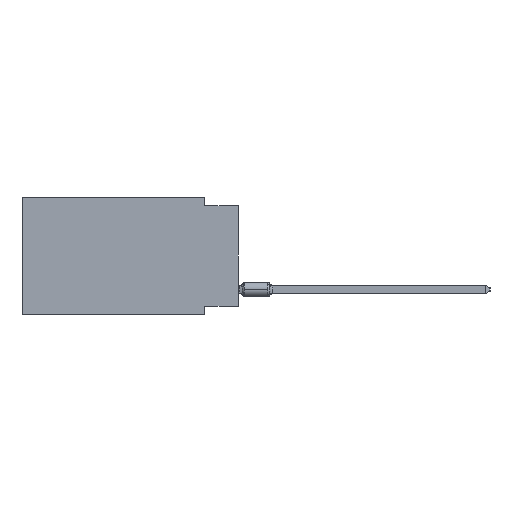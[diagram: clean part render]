
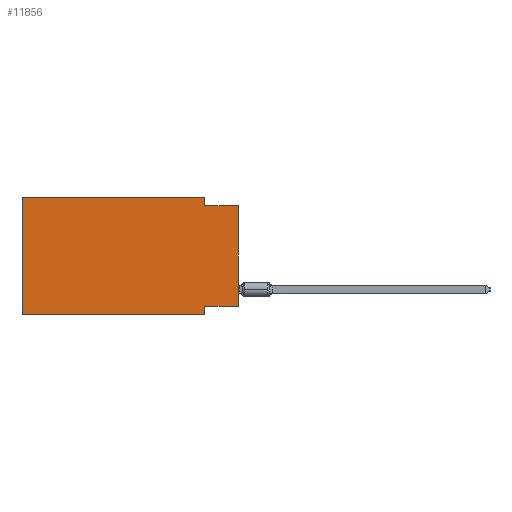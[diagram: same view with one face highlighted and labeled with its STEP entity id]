
A CAD part, left-side view. The second image highlights one B-rep face of the part: STEP entity #11856.
In plain terms, the highlighted planar face has unit normal (-1, 0, 0).
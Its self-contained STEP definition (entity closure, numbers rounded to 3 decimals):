
#1014 = EDGE_CURVE ( 'NONE', #4075, #43226, #54936, .T. ) ;
#1530 = CARTESIAN_POINT ( 'NONE',  ( 0., 2.54, -0.635 ) ) ;
#3191 = CARTESIAN_POINT ( 'NONE',  ( 0., 2.54, -8.255 ) ) ;
#4075 = VERTEX_POINT ( 'NONE', #3191 ) ;
#4749 = DIRECTION ( 'NONE',  ( 0., -1., 0. ) ) ;
#4871 = VECTOR ( 'NONE', #45037, 1000. ) ;
#9013 = VERTEX_POINT ( 'NONE', #46708 ) ;
#9141 = VERTEX_POINT ( 'NONE', #58113 ) ;
#9778 = LINE ( 'NONE', #30232, #64636 ) ;
#10782 = LINE ( 'NONE', #36605, #29411 ) ;
#11094 = DIRECTION ( 'NONE',  ( 0., 1., 0. ) ) ;
#11856 = ADVANCED_FACE ( 'NONE', ( #58854 ), #63882, .F. ) ;
#12960 = ORIENTED_EDGE ( 'NONE', *, *, #26854, .F. ) ;
#14326 = CARTESIAN_POINT ( 'NONE',  ( 0., 2.54, 0. ) ) ;
#17411 = ORIENTED_EDGE ( 'NONE', *, *, #57949, .T. ) ;
#19886 = AXIS2_PLACEMENT_3D ( 'NONE', #28637, #33326, #22628 ) ;
#19986 = LINE ( 'NONE', #25047, #54908 ) ;
#22628 = DIRECTION ( 'NONE',  ( 0., 0., -1. ) ) ;
#22693 = CARTESIAN_POINT ( 'NONE',  ( 0., 16.383, 0. ) ) ;
#24051 = ORIENTED_EDGE ( 'NONE', *, *, #45005, .F. ) ;
#25047 = CARTESIAN_POINT ( 'NONE',  ( 0., 0., -0.635 ) ) ;
#26339 = ORIENTED_EDGE ( 'NONE', *, *, #48039, .T. ) ;
#26854 = EDGE_CURVE ( 'NONE', #54475, #36489, #34770, .T. ) ;
#28362 = ORIENTED_EDGE ( 'NONE', *, *, #33851, .F. ) ;
#28637 = CARTESIAN_POINT ( 'NONE',  ( 0., 16.383, 0. ) ) ;
#29134 = EDGE_LOOP ( 'NONE', ( #26339, #41479, #12960, #24051, #28362, #17411, #55665, #57179 ) ) ;
#29411 = VECTOR ( 'NONE', #46338, 1000. ) ;
#30232 = CARTESIAN_POINT ( 'NONE',  ( 0., 16.383, 0. ) ) ;
#30508 = CARTESIAN_POINT ( 'NONE',  ( 0., 2.54, 0. ) ) ;
#31730 = LINE ( 'NONE', #52192, #57938 ) ;
#32688 = VERTEX_POINT ( 'NONE', #63521 ) ;
#33326 = DIRECTION ( 'NONE',  ( 1., 0., 0. ) ) ;
#33851 = EDGE_CURVE ( 'NONE', #9013, #9141, #39337, .T. ) ;
#34770 = LINE ( 'NONE', #14326, #40556 ) ;
#36489 = VERTEX_POINT ( 'NONE', #1530 ) ;
#36605 = CARTESIAN_POINT ( 'NONE',  ( 0., 0., 0. ) ) ;
#39337 = LINE ( 'NONE', #22693, #4871 ) ;
#40556 = VECTOR ( 'NONE', #42609, 1000. ) ;
#41479 = ORIENTED_EDGE ( 'NONE', *, *, #62569, .F. ) ;
#41804 = CARTESIAN_POINT ( 'NONE',  ( 0., 2.54, -8.89 ) ) ;
#42609 = DIRECTION ( 'NONE',  ( 0., 0., -1. ) ) ;
#43226 = VERTEX_POINT ( 'NONE', #41804 ) ;
#45005 = EDGE_CURVE ( 'NONE', #9141, #54475, #9778, .T. ) ;
#45037 = DIRECTION ( 'NONE',  ( 0., 0., 1. ) ) ;
#46240 = VECTOR ( 'NONE', #11094, 1000. ) ;
#46338 = DIRECTION ( 'NONE',  ( 0., 0., 1. ) ) ;
#46708 = CARTESIAN_POINT ( 'NONE',  ( 0., 16.383, -8.89 ) ) ;
#46877 = VECTOR ( 'NONE', #64346, 1000. ) ;
#48039 = EDGE_CURVE ( 'NONE', #32688, #51304, #10782, .T. ) ;
#48299 = DIRECTION ( 'NONE',  ( 0., -1., 0. ) ) ;
#49890 = CARTESIAN_POINT ( 'NONE',  ( 0., 2.54, -8.89 ) ) ;
#50139 = EDGE_CURVE ( 'NONE', #32688, #4075, #52006, .T. ) ;
#51304 = VERTEX_POINT ( 'NONE', #60676 ) ;
#52006 = LINE ( 'NONE', #52341, #46240 ) ;
#52192 = CARTESIAN_POINT ( 'NONE',  ( 0., 16.383, -8.89 ) ) ;
#52341 = CARTESIAN_POINT ( 'NONE',  ( 0., 0., -8.255 ) ) ;
#54475 = VERTEX_POINT ( 'NONE', #30508 ) ;
#54908 = VECTOR ( 'NONE', #48299, 1000. ) ;
#54936 = LINE ( 'NONE', #49890, #46877 ) ;
#55665 = ORIENTED_EDGE ( 'NONE', *, *, #1014, .F. ) ;
#57179 = ORIENTED_EDGE ( 'NONE', *, *, #50139, .F. ) ;
#57938 = VECTOR ( 'NONE', #58239, 1000. ) ;
#57949 = EDGE_CURVE ( 'NONE', #9013, #43226, #31730, .T. ) ;
#58113 = CARTESIAN_POINT ( 'NONE',  ( 0., 16.383, 0. ) ) ;
#58239 = DIRECTION ( 'NONE',  ( 0., -1., 0. ) ) ;
#58854 = FACE_OUTER_BOUND ( 'NONE', #29134, .T. ) ;
#60676 = CARTESIAN_POINT ( 'NONE',  ( 0., 0., -0.635 ) ) ;
#62569 = EDGE_CURVE ( 'NONE', #36489, #51304, #19986, .T. ) ;
#63521 = CARTESIAN_POINT ( 'NONE',  ( 0., 0., -8.255 ) ) ;
#63882 = PLANE ( 'NONE',  #19886 ) ;
#64346 = DIRECTION ( 'NONE',  ( 0., 0., -1. ) ) ;
#64636 = VECTOR ( 'NONE', #4749, 1000. ) ;
